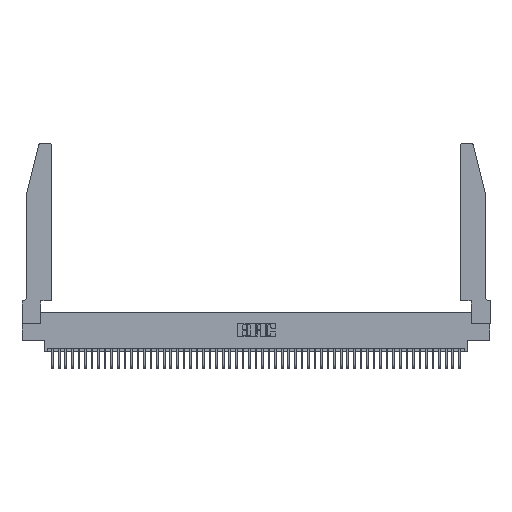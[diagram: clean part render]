
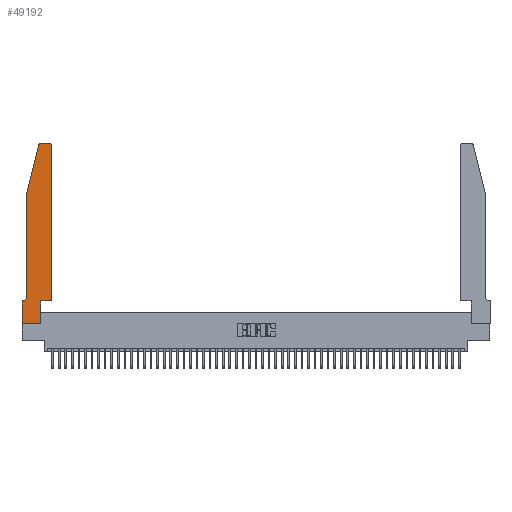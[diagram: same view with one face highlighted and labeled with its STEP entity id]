
A CAD part, top view. The second image highlights one B-rep face of the part: STEP entity #49192.
In plain terms, the highlighted planar face has unit normal (0, 0, 1).
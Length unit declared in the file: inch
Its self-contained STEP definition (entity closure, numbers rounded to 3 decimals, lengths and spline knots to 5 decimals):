
#512 = CIRCLE ( 'NONE', #9830, 0.03 ) ;
#2216 = DIRECTION ( 'NONE',  ( 0., 0., 1. ) ) ;
#2586 = ORIENTED_EDGE ( 'NONE', *, *, #14713, .T. ) ;
#2765 = DIRECTION ( 'NONE',  ( 1., 0., 0. ) ) ;
#2855 = VECTOR ( 'NONE', #6591, 39.37008 ) ;
#3039 = CARTESIAN_POINT ( 'NONE',  ( 0.4505, 0.35, 0.37 ) ) ;
#3066 = CARTESIAN_POINT ( 'NONE',  ( 0.2605, 2.75, 0.37 ) ) ;
#3495 = EDGE_CURVE ( 'NONE', #12042, #27451, #44790, .T. ) ;
#3832 = LINE ( 'NONE', #3039, #14007 ) ;
#4478 = CARTESIAN_POINT ( 'NONE',  ( 0., 0., 0.37 ) ) ;
#4488 = CARTESIAN_POINT ( 'NONE',  ( 0.2865, 0.35, 0.37 ) ) ;
#4525 = VERTEX_POINT ( 'NONE', #40655 ) ;
#6550 = AXIS2_PLACEMENT_3D ( 'NONE', #11264, #38115, #15142 ) ;
#6591 = DIRECTION ( 'NONE',  ( 0., -1., 0. ) ) ;
#6915 = DIRECTION ( 'NONE',  ( -1., 0., 0. ) ) ;
#6931 = VECTOR ( 'NONE', #23418, 39.37008 ) ;
#8262 = CARTESIAN_POINT ( 'NONE',  ( 0.284, 2.72, 0.37 ) ) ;
#8927 = CARTESIAN_POINT ( 'NONE',  ( 0.0755, 0.42, 0.37 ) ) ;
#9830 = AXIS2_PLACEMENT_3D ( 'NONE', #25204, #2216, #29102 ) ;
#11023 = VERTEX_POINT ( 'NONE', #16087 ) ;
#11264 = CARTESIAN_POINT ( 'NONE',  ( 0.0055, 0.42, 0.37 ) ) ;
#11679 = ORIENTED_EDGE ( 'NONE', *, *, #28233, .T. ) ;
#11954 = CARTESIAN_POINT ( 'NONE',  ( 0.284, 2.75, 0.37 ) ) ;
#12042 = VERTEX_POINT ( 'NONE', #49049 ) ;
#12123 = DIRECTION ( 'NONE',  ( 1., 0., 0. ) ) ;
#12756 = EDGE_CURVE ( 'NONE', #20783, #11023, #41836, .T. ) ;
#14007 = VECTOR ( 'NONE', #22164, 39.37008 ) ;
#14713 = EDGE_CURVE ( 'NONE', #15322, #28822, #16254, .T. ) ;
#15142 = DIRECTION ( 'NONE',  ( -1., 0., 0. ) ) ;
#15322 = VERTEX_POINT ( 'NONE', #18278 ) ;
#15488 = LINE ( 'NONE', #4488, #23269 ) ;
#15950 = ORIENTED_EDGE ( 'NONE', *, *, #34288, .T. ) ;
#16087 = CARTESIAN_POINT ( 'NONE',  ( 0.2865, 0., 0.37 ) ) ;
#16254 = LINE ( 'NONE', #3066, #41998 ) ;
#16572 = EDGE_CURVE ( 'NONE', #34470, #15322, #512, .T. ) ;
#16971 = VERTEX_POINT ( 'NONE', #40406 ) ;
#17087 = ORIENTED_EDGE ( 'NONE', *, *, #24268, .T. ) ;
#17335 = LINE ( 'NONE', #4478, #18544 ) ;
#17901 = VECTOR ( 'NONE', #48539, 39.37008 ) ;
#18278 = CARTESIAN_POINT ( 'NONE',  ( 0.4205, 2.75, 0.37 ) ) ;
#18544 = VECTOR ( 'NONE', #31369, 39.37008 ) ;
#19093 = LINE ( 'NONE', #21856, #17901 ) ;
#19295 = CARTESIAN_POINT ( 'NONE',  ( 0.4505, 2.72, 0.37 ) ) ;
#19454 = DIRECTION ( 'NONE',  ( 1., 0., 0. ) ) ;
#20783 = VERTEX_POINT ( 'NONE', #28498 ) ;
#21498 = VECTOR ( 'NONE', #19454, 39.37008 ) ;
#21856 = CARTESIAN_POINT ( 'NONE',  ( 0.0755, 2., 0.37 ) ) ;
#22164 = DIRECTION ( 'NONE',  ( 1., 0., 0. ) ) ;
#22382 = EDGE_CURVE ( 'NONE', #4525, #27765, #47609, .T. ) ;
#23269 = VECTOR ( 'NONE', #23600, 39.37008 ) ;
#23418 = DIRECTION ( 'NONE',  ( -1., 0., 0. ) ) ;
#23600 = DIRECTION ( 'NONE',  ( 0., 1., 0. ) ) ;
#24268 = EDGE_CURVE ( 'NONE', #27451, #4525, #43866, .T. ) ;
#25204 = CARTESIAN_POINT ( 'NONE',  ( 0.4205, 2.72, 0.37 ) ) ;
#25724 = CARTESIAN_POINT ( 'NONE',  ( 0.0755, 2., 0.37 ) ) ;
#25754 = DIRECTION ( 'NONE',  ( 0., 0., 1. ) ) ;
#26398 = CARTESIAN_POINT ( 'NONE',  ( 0., 0.35, 0.37 ) ) ;
#27451 = VERTEX_POINT ( 'NONE', #8927 ) ;
#27765 = VERTEX_POINT ( 'NONE', #26398 ) ;
#27938 = ORIENTED_EDGE ( 'NONE', *, *, #22382, .T. ) ;
#28233 = EDGE_CURVE ( 'NONE', #11023, #33421, #15488, .T. ) ;
#28498 = CARTESIAN_POINT ( 'NONE',  ( 0., 0., 0.37 ) ) ;
#28822 = VERTEX_POINT ( 'NONE', #11954 ) ;
#29102 = DIRECTION ( 'NONE',  ( 1., 0., 0. ) ) ;
#29285 = ORIENTED_EDGE ( 'NONE', *, *, #16572, .T. ) ;
#29672 = CARTESIAN_POINT ( 'NONE',  ( 0.4505, 0.35, 0.37 ) ) ;
#29812 = ORIENTED_EDGE ( 'NONE', *, *, #47956, .T. ) ;
#30003 = DIRECTION ( 'NONE',  ( 0., 1., 0. ) ) ;
#30468 = CARTESIAN_POINT ( 'NONE',  ( 0.2865, 0.35, 0.37 ) ) ;
#31369 = DIRECTION ( 'NONE',  ( 0., -1., 0. ) ) ;
#32087 = ORIENTED_EDGE ( 'NONE', *, *, #3495, .T. ) ;
#33421 = VERTEX_POINT ( 'NONE', #30468 ) ;
#33670 = AXIS2_PLACEMENT_3D ( 'NONE', #48421, #25754, #2765 ) ;
#33841 = ORIENTED_EDGE ( 'NONE', *, *, #44842, .T. ) ;
#34288 = EDGE_CURVE ( 'NONE', #33421, #43917, #3832, .T. ) ;
#34470 = VERTEX_POINT ( 'NONE', #19295 ) ;
#35003 = CARTESIAN_POINT ( 'NONE',  ( 0.4505, 0.35, 0.37 ) ) ;
#35014 = CARTESIAN_POINT ( 'NONE',  ( 0.0755, 0.35, 0.37 ) ) ;
#35147 = DIRECTION ( 'NONE',  ( 0., 0., 1. ) ) ;
#35378 = VECTOR ( 'NONE', #30003, 39.37008 ) ;
#37148 = EDGE_CURVE ( 'NONE', #28822, #16971, #43142, .T. ) ;
#38115 = DIRECTION ( 'NONE',  ( 0., 0., -1. ) ) ;
#40406 = CARTESIAN_POINT ( 'NONE',  ( 0.25487, 2.72718, 0.37 ) ) ;
#40655 = CARTESIAN_POINT ( 'NONE',  ( 0.0055, 0.35, 0.37 ) ) ;
#41580 = AXIS2_PLACEMENT_3D ( 'NONE', #8262, #35147, #12123 ) ;
#41594 = EDGE_LOOP ( 'NONE', ( #2586, #46872, #33841, #32087, #17087, #27938, #45825, #47634, #11679, #15950, #29812, #29285 ) ) ;
#41836 = LINE ( 'NONE', #42375, #21498 ) ;
#41998 = VECTOR ( 'NONE', #6915, 39.37008 ) ;
#42375 = CARTESIAN_POINT ( 'NONE',  ( 0., 0., 0.37 ) ) ;
#43142 = CIRCLE ( 'NONE', #41580, 0.03 ) ;
#43866 = CIRCLE ( 'NONE', #6550, 0.07 ) ;
#43917 = VERTEX_POINT ( 'NONE', #35003 ) ;
#44790 = LINE ( 'NONE', #25724, #2855 ) ;
#44842 = EDGE_CURVE ( 'NONE', #16971, #12042, #19093, .T. ) ;
#45825 = ORIENTED_EDGE ( 'NONE', *, *, #47656, .T. ) ;
#46506 = FACE_OUTER_BOUND ( 'NONE', #41594, .T. ) ;
#46657 = LINE ( 'NONE', #29672, #35378 ) ;
#46872 = ORIENTED_EDGE ( 'NONE', *, *, #37148, .T. ) ;
#47609 = LINE ( 'NONE', #35014, #6931 ) ;
#47634 = ORIENTED_EDGE ( 'NONE', *, *, #12756, .T. ) ;
#47656 = EDGE_CURVE ( 'NONE', #27765, #20783, #17335, .T. ) ;
#47956 = EDGE_CURVE ( 'NONE', #43917, #34470, #46657, .T. ) ;
#48421 = CARTESIAN_POINT ( 'NONE',  ( 0., 0.35, 0.37 ) ) ;
#48539 = DIRECTION ( 'NONE',  ( -0.239, -0.971, 0. ) ) ;
#48582 = PLANE ( 'NONE',  #33670 ) ;
#49049 = CARTESIAN_POINT ( 'NONE',  ( 0.0755, 2., 0.37 ) ) ;
#49192 = ADVANCED_FACE ( 'NONE', ( #46506 ), #48582, .T. ) ;
